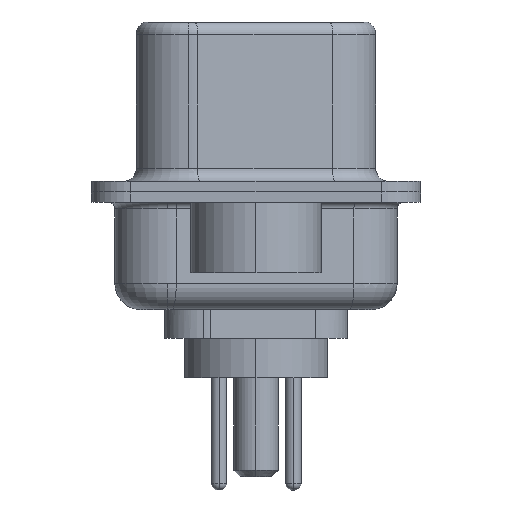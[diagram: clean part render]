
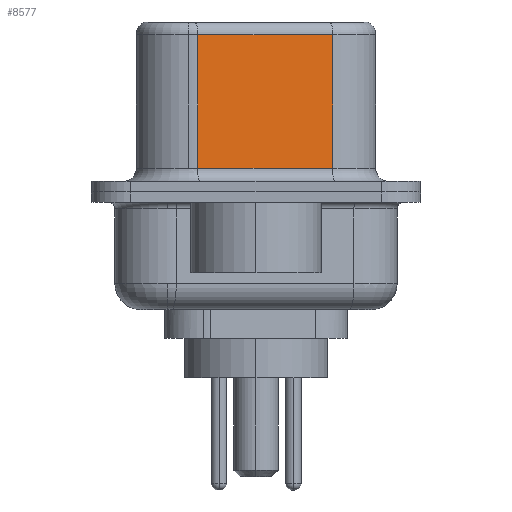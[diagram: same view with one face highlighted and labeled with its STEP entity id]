
A CAD part, left-side view. The second image highlights one B-rep face of the part: STEP entity #8577.
In plain terms, the highlighted planar face has unit normal (-0.985, -0.174, 0).
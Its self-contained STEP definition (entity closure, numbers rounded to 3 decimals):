
#782 = DIRECTION ( 'NONE',  ( 0., 0., -1. ) ) ;
#962 = PLANE ( 'NONE',  #18101 ) ;
#1659 = EDGE_LOOP ( 'NONE', ( #6216, #18054, #6228, #10591 ) ) ;
#4457 = CARTESIAN_POINT ( 'NONE',  ( 4.585, -2.927, 6.02 ) ) ;
#4951 = VERTEX_POINT ( 'NONE', #12190 ) ;
#6029 = EDGE_CURVE ( 'NONE', #17353, #4951, #14535, .T. ) ;
#6216 = ORIENTED_EDGE ( 'NONE', *, *, #6815, .F. ) ;
#6228 = ORIENTED_EDGE ( 'NONE', *, *, #6029, .T. ) ;
#6536 = VECTOR ( 'NONE', #782, 1000. ) ;
#6762 = FACE_OUTER_BOUND ( 'NONE', #1659, .T. ) ;
#6815 = EDGE_CURVE ( 'NONE', #17164, #13396, #14561, .T. ) ;
#7120 = DIRECTION ( 'NONE',  ( 0.174, -0.985, 0. ) ) ;
#7519 = DIRECTION ( 'NONE',  ( 0., 0., -1. ) ) ;
#8017 = CARTESIAN_POINT ( 'NONE',  ( 4.585, -2.927, 6.52 ) ) ;
#8577 = ADVANCED_FACE ( 'NONE', ( #6762 ), #962, .F. ) ;
#8730 = EDGE_CURVE ( 'NONE', #4951, #13396, #10070, .T. ) ;
#9184 = CARTESIAN_POINT ( 'NONE',  ( 4.585, -2.927, 6.02 ) ) ;
#9618 = VECTOR ( 'NONE', #7519, 1000. ) ;
#10070 = LINE ( 'NONE', #19332, #12854 ) ;
#10591 = ORIENTED_EDGE ( 'NONE', *, *, #8730, .T. ) ;
#11250 = CARTESIAN_POINT ( 'NONE',  ( 3.675, 2.233, 6.52 ) ) ;
#11376 = DIRECTION ( 'NONE',  ( 0.985, 0.174, 0. ) ) ;
#11445 = DIRECTION ( 'NONE',  ( -0.174, 0.985, 0. ) ) ;
#11688 = EDGE_CURVE ( 'NONE', #17164, #17353, #16984, .T. ) ;
#12190 = CARTESIAN_POINT ( 'NONE',  ( 3.675, 2.233, 0.9 ) ) ;
#12508 = VECTOR ( 'NONE', #14988, 1000. ) ;
#12854 = VECTOR ( 'NONE', #7120, 1000. ) ;
#13396 = VERTEX_POINT ( 'NONE', #16590 ) ;
#13782 = CARTESIAN_POINT ( 'NONE',  ( 3.675, 2.233, 6.02 ) ) ;
#14535 = LINE ( 'NONE', #11250, #6536 ) ;
#14561 = LINE ( 'NONE', #16449, #9618 ) ;
#14988 = DIRECTION ( 'NONE',  ( -0.174, 0.985, 0. ) ) ;
#16449 = CARTESIAN_POINT ( 'NONE',  ( 4.585, -2.927, 6.52 ) ) ;
#16590 = CARTESIAN_POINT ( 'NONE',  ( 4.585, -2.927, 0.9 ) ) ;
#16984 = LINE ( 'NONE', #4457, #12508 ) ;
#17164 = VERTEX_POINT ( 'NONE', #9184 ) ;
#17353 = VERTEX_POINT ( 'NONE', #13782 ) ;
#18054 = ORIENTED_EDGE ( 'NONE', *, *, #11688, .T. ) ;
#18101 = AXIS2_PLACEMENT_3D ( 'NONE', #8017, #11376, #11445 ) ;
#19332 = CARTESIAN_POINT ( 'NONE',  ( 4.585, -2.927, 0.9 ) ) ;
